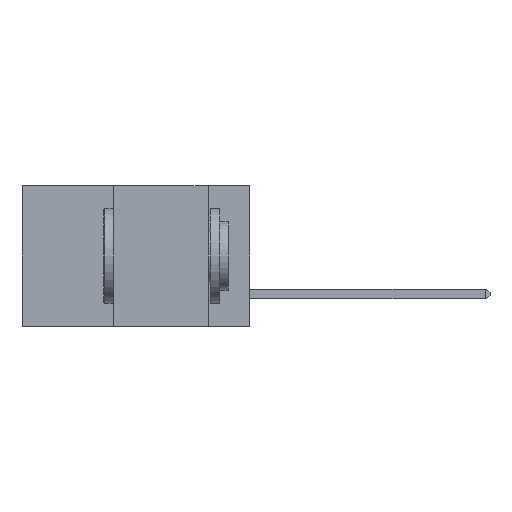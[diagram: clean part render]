
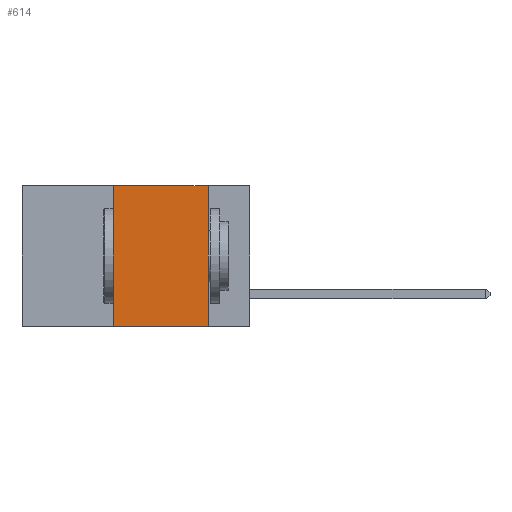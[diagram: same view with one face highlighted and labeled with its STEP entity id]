
A CAD part, left-side view. The second image highlights one B-rep face of the part: STEP entity #614.
In plain terms, the highlighted planar face has unit normal (-1, 0, 0).
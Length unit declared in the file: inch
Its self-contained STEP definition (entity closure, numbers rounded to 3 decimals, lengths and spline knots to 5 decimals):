
#436 = LINE ( 'NONE', #4478, #4129 ) ;
#614 = ADVANCED_FACE ( 'NONE', ( #10867 ), #777, .F. ) ;
#679 = CARTESIAN_POINT ( 'NONE',  ( 0., 0.11, -0.37 ) ) ;
#777 = PLANE ( 'NONE',  #3191 ) ;
#967 = CARTESIAN_POINT ( 'NONE',  ( 0., 0.36, -0.37 ) ) ;
#2498 = DIRECTION ( 'NONE',  ( 0., 0., -1. ) ) ;
#2537 = DIRECTION ( 'NONE',  ( 1., 0., 0. ) ) ;
#2561 = VECTOR ( 'NONE', #19639, 39.37008 ) ;
#2668 = ORIENTED_EDGE ( 'NONE', *, *, #11283, .F. ) ;
#3082 = LINE ( 'NONE', #8226, #10960 ) ;
#3191 = AXIS2_PLACEMENT_3D ( 'NONE', #3698, #2537, #2498 ) ;
#3649 = DIRECTION ( 'NONE',  ( 0., -1., 0. ) ) ;
#3698 = CARTESIAN_POINT ( 'NONE',  ( 0., 0.6, 0. ) ) ;
#4129 = VECTOR ( 'NONE', #3649, 39.37008 ) ;
#4415 = EDGE_CURVE ( 'NONE', #8263, #14123, #436, .T. ) ;
#4478 = CARTESIAN_POINT ( 'NONE',  ( 0., 0.6, 0. ) ) ;
#4511 = DIRECTION ( 'NONE',  ( 0., 0., -1. ) ) ;
#5188 = VERTEX_POINT ( 'NONE', #967 ) ;
#6994 = EDGE_LOOP ( 'NONE', ( #2668, #10738, #14931, #18899 ) ) ;
#7056 = EDGE_CURVE ( 'NONE', #5188, #10985, #11416, .T. ) ;
#8226 = CARTESIAN_POINT ( 'NONE',  ( 0., 0.36, 0. ) ) ;
#8263 = VERTEX_POINT ( 'NONE', #8893 ) ;
#8893 = CARTESIAN_POINT ( 'NONE',  ( 0., 0.36, 0. ) ) ;
#8981 = CARTESIAN_POINT ( 'NONE',  ( 0., 0.6, -0.37 ) ) ;
#10738 = ORIENTED_EDGE ( 'NONE', *, *, #4415, .F. ) ;
#10864 = CARTESIAN_POINT ( 'NONE',  ( 0., 0.11, 0. ) ) ;
#10867 = FACE_OUTER_BOUND ( 'NONE', #6994, .T. ) ;
#10960 = VECTOR ( 'NONE', #18954, 39.37008 ) ;
#10985 = VERTEX_POINT ( 'NONE', #679 ) ;
#11283 = EDGE_CURVE ( 'NONE', #14123, #10985, #19237, .T. ) ;
#11416 = LINE ( 'NONE', #8981, #2561 ) ;
#11859 = CARTESIAN_POINT ( 'NONE',  ( 0., 0.11, 0. ) ) ;
#14123 = VERTEX_POINT ( 'NONE', #11859 ) ;
#14931 = ORIENTED_EDGE ( 'NONE', *, *, #17032, .F. ) ;
#15273 = VECTOR ( 'NONE', #4511, 39.37008 ) ;
#17032 = EDGE_CURVE ( 'NONE', #5188, #8263, #3082, .T. ) ;
#18899 = ORIENTED_EDGE ( 'NONE', *, *, #7056, .T. ) ;
#18954 = DIRECTION ( 'NONE',  ( 0., 0., 1. ) ) ;
#19237 = LINE ( 'NONE', #10864, #15273 ) ;
#19639 = DIRECTION ( 'NONE',  ( 0., -1., 0. ) ) ;
